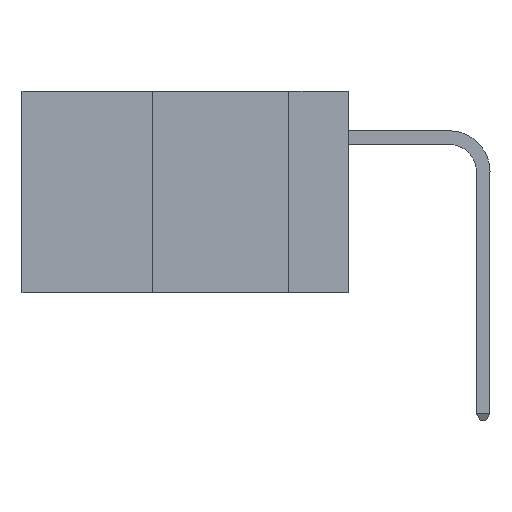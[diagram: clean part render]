
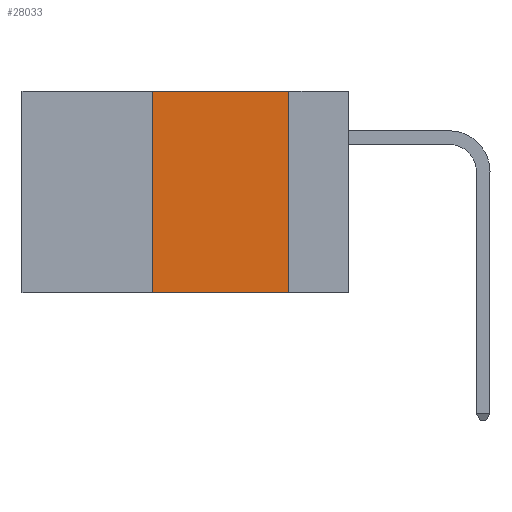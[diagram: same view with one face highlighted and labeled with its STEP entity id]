
A CAD part, left-side view. The second image highlights one B-rep face of the part: STEP entity #28033.
In plain terms, the highlighted planar face has unit normal (-1, 0, 0).
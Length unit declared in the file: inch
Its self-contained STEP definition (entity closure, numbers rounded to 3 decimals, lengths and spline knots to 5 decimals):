
#328 = VECTOR ( 'NONE', #28276, 39.37008 ) ;
#816 = VECTOR ( 'NONE', #15356, 39.37008 ) ;
#1062 = CARTESIAN_POINT ( 'NONE',  ( 0., 0.6, -0.37 ) ) ;
#1795 = LINE ( 'NONE', #8726, #20208 ) ;
#1979 = LINE ( 'NONE', #1062, #816 ) ;
#5239 = FACE_OUTER_BOUND ( 'NONE', #15473, .T. ) ;
#5797 = ORIENTED_EDGE ( 'NONE', *, *, #17354, .F. ) ;
#6721 = LINE ( 'NONE', #21017, #328 ) ;
#7215 = VERTEX_POINT ( 'NONE', #30903 ) ;
#8726 = CARTESIAN_POINT ( 'NONE',  ( 0., 0.11, 0. ) ) ;
#8959 = DIRECTION ( 'NONE',  ( 0., 0., -1. ) ) ;
#10055 = AXIS2_PLACEMENT_3D ( 'NONE', #13825, #23372, #8959 ) ;
#11585 = EDGE_CURVE ( 'NONE', #15349, #27144, #1795, .T. ) ;
#11597 = PLANE ( 'NONE',  #10055 ) ;
#13344 = CARTESIAN_POINT ( 'NONE',  ( 0., 0.36, -0.37 ) ) ;
#13825 = CARTESIAN_POINT ( 'NONE',  ( 0., 0.6, 0. ) ) ;
#13946 = LINE ( 'NONE', #29032, #21092 ) ;
#15349 = VERTEX_POINT ( 'NONE', #17745 ) ;
#15356 = DIRECTION ( 'NONE',  ( 0., -1., 0. ) ) ;
#15473 = EDGE_LOOP ( 'NONE', ( #20168, #21230, #5797, #29099 ) ) ;
#17354 = EDGE_CURVE ( 'NONE', #28624, #7215, #6721, .T. ) ;
#17745 = CARTESIAN_POINT ( 'NONE',  ( 0., 0.11, 0. ) ) ;
#20168 = ORIENTED_EDGE ( 'NONE', *, *, #11585, .F. ) ;
#20208 = VECTOR ( 'NONE', #25575, 39.37008 ) ;
#21017 = CARTESIAN_POINT ( 'NONE',  ( 0., 0.36, 0. ) ) ;
#21092 = VECTOR ( 'NONE', #26394, 39.37008 ) ;
#21230 = ORIENTED_EDGE ( 'NONE', *, *, #28794, .F. ) ;
#22067 = CARTESIAN_POINT ( 'NONE',  ( 0., 0.11, -0.37 ) ) ;
#23372 = DIRECTION ( 'NONE',  ( 1., 0., 0. ) ) ;
#25575 = DIRECTION ( 'NONE',  ( 0., 0., -1. ) ) ;
#25705 = EDGE_CURVE ( 'NONE', #28624, #27144, #1979, .T. ) ;
#26394 = DIRECTION ( 'NONE',  ( 0., -1., 0. ) ) ;
#27144 = VERTEX_POINT ( 'NONE', #22067 ) ;
#28033 = ADVANCED_FACE ( 'NONE', ( #5239 ), #11597, .F. ) ;
#28276 = DIRECTION ( 'NONE',  ( 0., 0., 1. ) ) ;
#28624 = VERTEX_POINT ( 'NONE', #13344 ) ;
#28794 = EDGE_CURVE ( 'NONE', #7215, #15349, #13946, .T. ) ;
#29032 = CARTESIAN_POINT ( 'NONE',  ( 0., 0.6, 0. ) ) ;
#29099 = ORIENTED_EDGE ( 'NONE', *, *, #25705, .T. ) ;
#30903 = CARTESIAN_POINT ( 'NONE',  ( 0., 0.36, 0. ) ) ;
